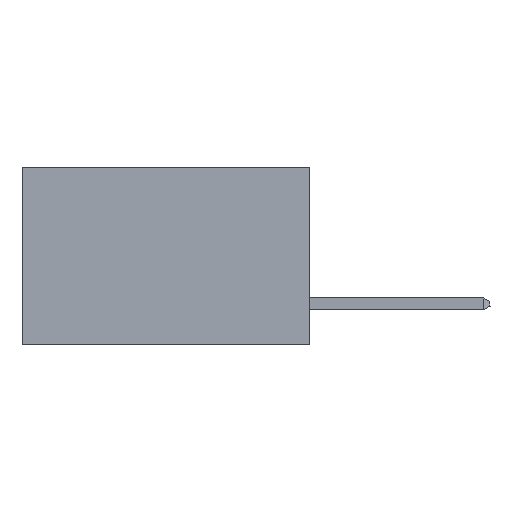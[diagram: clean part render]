
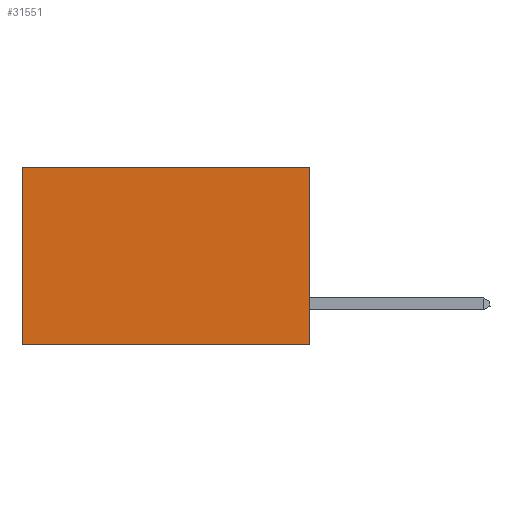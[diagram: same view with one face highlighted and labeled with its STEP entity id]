
A CAD part, left-side view. The second image highlights one B-rep face of the part: STEP entity #31551.
In plain terms, the highlighted planar face has unit normal (-1, 0, 0).
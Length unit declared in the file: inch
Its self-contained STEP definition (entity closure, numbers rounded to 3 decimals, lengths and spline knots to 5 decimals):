
#96 = DIRECTION ( 'NONE',  ( 0., 0., -1. ) ) ;
#612 = VECTOR ( 'NONE', #23752, 39.37008 ) ;
#1431 = VECTOR ( 'NONE', #7370, 39.37008 ) ;
#2488 = ORIENTED_EDGE ( 'NONE', *, *, #28886, .F. ) ;
#2935 = VERTEX_POINT ( 'NONE', #36119 ) ;
#5479 = VECTOR ( 'NONE', #32310, 39.37008 ) ;
#5757 = CARTESIAN_POINT ( 'NONE',  ( 0.2875, 0.6, 0. ) ) ;
#6913 = LINE ( 'NONE', #34295, #17401 ) ;
#7290 = EDGE_LOOP ( 'NONE', ( #14276, #2488, #29420, #15465 ) ) ;
#7370 = DIRECTION ( 'NONE',  ( 0., 1., 0. ) ) ;
#12207 = DIRECTION ( 'NONE',  ( 1., 0., 0. ) ) ;
#12882 = DIRECTION ( 'NONE',  ( 0., 0., -1. ) ) ;
#14276 = ORIENTED_EDGE ( 'NONE', *, *, #27307, .T. ) ;
#15465 = ORIENTED_EDGE ( 'NONE', *, *, #22344, .T. ) ;
#17401 = VECTOR ( 'NONE', #12882, 39.37008 ) ;
#18331 = PLANE ( 'NONE',  #36785 ) ;
#21675 = LINE ( 'NONE', #26322, #5479 ) ;
#22344 = EDGE_CURVE ( 'NONE', #31190, #34345, #21675, .T. ) ;
#22688 = CARTESIAN_POINT ( 'NONE',  ( 0.2875, 0., -0.37 ) ) ;
#23752 = DIRECTION ( 'NONE',  ( 0., 0., -1. ) ) ;
#23911 = FACE_OUTER_BOUND ( 'NONE', #7290, .T. ) ;
#24170 = CARTESIAN_POINT ( 'NONE',  ( 0.2875, 0., 0. ) ) ;
#24861 = LINE ( 'NONE', #5757, #612 ) ;
#25130 = EDGE_CURVE ( 'NONE', #31190, #2935, #6913, .T. ) ;
#26002 = CARTESIAN_POINT ( 'NONE',  ( 0.2875, 0.6, -0.37 ) ) ;
#26322 = CARTESIAN_POINT ( 'NONE',  ( 0.2875, 0., 0. ) ) ;
#27307 = EDGE_CURVE ( 'NONE', #34345, #35357, #24861, .T. ) ;
#27550 = LINE ( 'NONE', #22688, #1431 ) ;
#28886 = EDGE_CURVE ( 'NONE', #2935, #35357, #27550, .T. ) ;
#29420 = ORIENTED_EDGE ( 'NONE', *, *, #25130, .F. ) ;
#29802 = CARTESIAN_POINT ( 'NONE',  ( 0.2875, 0.6, 0. ) ) ;
#31190 = VERTEX_POINT ( 'NONE', #32037 ) ;
#31551 = ADVANCED_FACE ( 'NONE', ( #23911 ), #18331, .F. ) ;
#32037 = CARTESIAN_POINT ( 'NONE',  ( 0.2875, 0., 0. ) ) ;
#32310 = DIRECTION ( 'NONE',  ( 0., 1., 0. ) ) ;
#34295 = CARTESIAN_POINT ( 'NONE',  ( 0.2875, 0., 0. ) ) ;
#34345 = VERTEX_POINT ( 'NONE', #29802 ) ;
#35357 = VERTEX_POINT ( 'NONE', #26002 ) ;
#36119 = CARTESIAN_POINT ( 'NONE',  ( 0.2875, 0., -0.37 ) ) ;
#36785 = AXIS2_PLACEMENT_3D ( 'NONE', #24170, #12207, #96 ) ;
